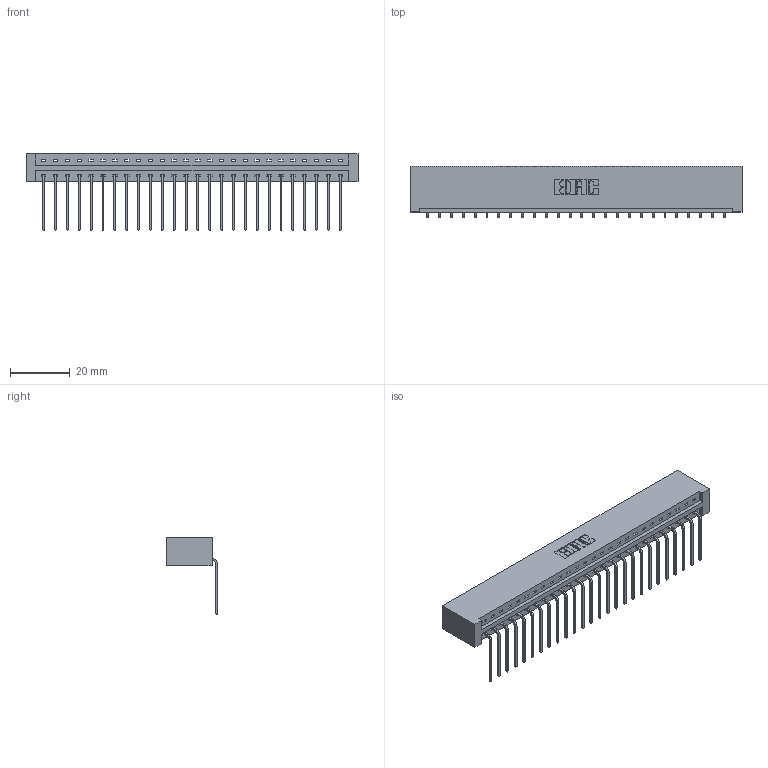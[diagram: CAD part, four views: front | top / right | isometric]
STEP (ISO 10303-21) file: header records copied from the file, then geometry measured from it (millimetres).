
FILE_DESCRIPTION (( 'STEP AP203' ), '1' );
FILE_NAME ('337-026-559-101.STEP', '2018-08-06T06:37:08', ( '' ), ( '' ), 'SwSTEP 2.0', 'SolidWorks 2016', '' );
FILE_SCHEMA (( 'CONFIG_CONTROL_DESIGN' ));
Length unit declared in the file: inch
Products named in the file (3): 337 Part_No Mounting Lugs; 345-292-001_558 559 Tail - 1; 337-026-559-101
Assembly tree (27 placements, depth 2):
  337-026-559-101
    337 Part_No Mounting Lugs
    345-292-001_558 559 Tail - 1  x26
Bounding box: 110.9 x 17.09 x 25.53 mm (x, y, z)
Volume: 12150.9 mm3; surface area: 12981 mm2
Topology: 27 solids, 27 shells, 1770 faces, 5331 edges, 3518 vertices
Faces by surface type: plane 1314, cylinder 456
Entity records: 21203 total; most frequent: CARTESIAN_POINT 3700, ORIENTED_EDGE 3662, DIRECTION 3139, EDGE_CURVE 1831, LINE 1711, VECTOR 1711, VERTEX_POINT 1218, AXIS2_PLACEMENT_3D 714
